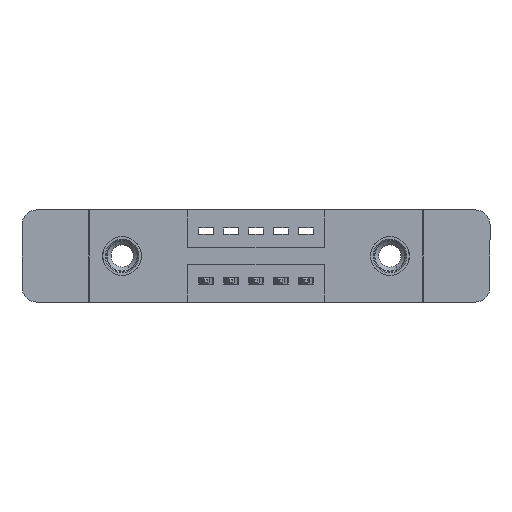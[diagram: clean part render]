
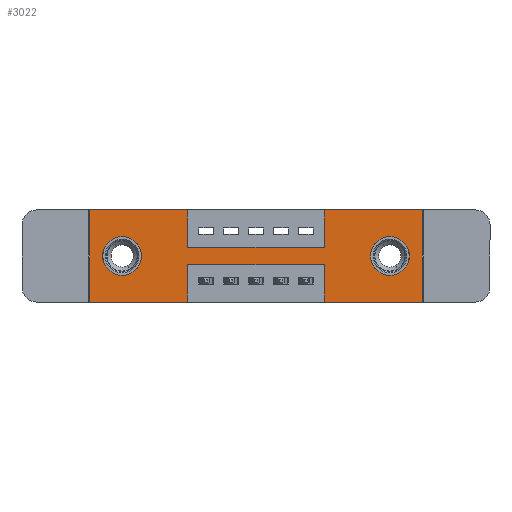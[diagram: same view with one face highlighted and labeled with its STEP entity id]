
A CAD part, front view. The second image highlights one B-rep face of the part: STEP entity #3022.
In plain terms, the highlighted planar face has unit normal (0, -1, 0).
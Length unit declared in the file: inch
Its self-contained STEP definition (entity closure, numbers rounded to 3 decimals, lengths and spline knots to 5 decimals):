
#40 = VECTOR ( 'NONE', #10457, 39.37008 ) ;
#335 = AXIS2_PLACEMENT_3D ( 'NONE', #2708, #11473, #4994 ) ;
#441 = VECTOR ( 'NONE', #3727, 39.37008 ) ;
#442 = VECTOR ( 'NONE', #2713, 39.37008 ) ;
#696 = EDGE_CURVE ( 'NONE', #11015, #10530, #4663, .T. ) ;
#732 = ORIENTED_EDGE ( 'NONE', *, *, #8910, .F. ) ;
#839 = LINE ( 'NONE', #7332, #11649 ) ;
#999 = CARTESIAN_POINT ( 'NONE',  ( 0., 0., -0.37 ) ) ;
#1172 = VECTOR ( 'NONE', #13573, 39.37008 ) ;
#1231 = EDGE_CURVE ( 'NONE', #11217, #7812, #3303, .T. ) ;
#1261 = VERTEX_POINT ( 'NONE', #6042 ) ;
#1301 = VERTEX_POINT ( 'NONE', #3097 ) ;
#1337 = ORIENTED_EDGE ( 'NONE', *, *, #5611, .F. ) ;
#1374 = CARTESIAN_POINT ( 'NONE',  ( 0.13, 0., -0.185 ) ) ;
#1427 = AXIS2_PLACEMENT_3D ( 'NONE', #5837, #6946, #1541 ) ;
#1432 = LINE ( 'NONE', #1782, #7557 ) ;
#1444 = LINE ( 'NONE', #6855, #441 ) ;
#1499 = DIRECTION ( 'NONE',  ( 0., 0., -1. ) ) ;
#1541 = DIRECTION ( 'NONE',  ( 0., 0., 1. ) ) ;
#1595 = DIRECTION ( 'NONE',  ( 0., 1., 0. ) ) ;
#1655 = EDGE_LOOP ( 'NONE', ( #13437, #12144, #732, #12489, #5523, #8941, #12088, #11838, #7246, #10654, #1337, #10598 ) ) ;
#1717 = VERTEX_POINT ( 'NONE', #11412 ) ;
#1782 = CARTESIAN_POINT ( 'NONE',  ( 0., 0., -0.37 ) ) ;
#2211 = LINE ( 'NONE', #9366, #40 ) ;
#2405 = CARTESIAN_POINT ( 'NONE',  ( 1.335, 0., 0. ) ) ;
#2530 = DIRECTION ( 'NONE',  ( 1., 0., 0. ) ) ;
#2640 = CARTESIAN_POINT ( 'NONE',  ( 0., 0., 0. ) ) ;
#2665 = ORIENTED_EDGE ( 'NONE', *, *, #8342, .T. ) ;
#2708 = CARTESIAN_POINT ( 'NONE',  ( 1.205, 0., -0.185 ) ) ;
#2713 = DIRECTION ( 'NONE',  ( 0., 0., -1. ) ) ;
#2794 = CARTESIAN_POINT ( 'NONE',  ( 1.335, 0., 0. ) ) ;
#2797 = VECTOR ( 'NONE', #5978, 39.37008 ) ;
#2984 = CIRCLE ( 'NONE', #1427, 0.078 ) ;
#3022 = ADVANCED_FACE ( 'NONE', ( #10549, #8697, #5294 ), #7953, .T. ) ;
#3045 = DIRECTION ( 'NONE',  ( -1., 0., 0. ) ) ;
#3097 = CARTESIAN_POINT ( 'NONE',  ( 0.13, 0., -0.263 ) ) ;
#3152 = CARTESIAN_POINT ( 'NONE',  ( 0.3925, 0., -0.15 ) ) ;
#3303 = LINE ( 'NONE', #7256, #442 ) ;
#3496 = CARTESIAN_POINT ( 'NONE',  ( 0., 0., 0. ) ) ;
#3504 = DIRECTION ( 'NONE',  ( 0., 0., 1. ) ) ;
#3627 = DIRECTION ( 'NONE',  ( 0., -1., 0. ) ) ;
#3727 = DIRECTION ( 'NONE',  ( 0., 0., 1. ) ) ;
#3757 = EDGE_CURVE ( 'NONE', #1717, #11015, #2211, .T. ) ;
#3911 = VERTEX_POINT ( 'NONE', #5735 ) ;
#4175 = CIRCLE ( 'NONE', #9367, 0.078 ) ;
#4194 = VERTEX_POINT ( 'NONE', #3496 ) ;
#4247 = CIRCLE ( 'NONE', #335, 0.078 ) ;
#4253 = VERTEX_POINT ( 'NONE', #9760 ) ;
#4655 = CARTESIAN_POINT ( 'NONE',  ( 0.3925, 0., 0. ) ) ;
#4663 = LINE ( 'NONE', #2640, #2797 ) ;
#4710 = CARTESIAN_POINT ( 'NONE',  ( 0., 0., -0.37 ) ) ;
#4851 = ORIENTED_EDGE ( 'NONE', *, *, #12152, .T. ) ;
#4985 = LINE ( 'NONE', #5798, #10904 ) ;
#4994 = DIRECTION ( 'NONE',  ( 0., 0., -1. ) ) ;
#5043 = EDGE_CURVE ( 'NONE', #12837, #11812, #12834, .T. ) ;
#5129 = EDGE_CURVE ( 'NONE', #4194, #12837, #5736, .T. ) ;
#5294 = FACE_OUTER_BOUND ( 'NONE', #1655, .T. ) ;
#5468 = CARTESIAN_POINT ( 'NONE',  ( 0.9425, 0., -0.22 ) ) ;
#5523 = ORIENTED_EDGE ( 'NONE', *, *, #10918, .F. ) ;
#5611 = EDGE_CURVE ( 'NONE', #9312, #4194, #10639, .T. ) ;
#5660 = CARTESIAN_POINT ( 'NONE',  ( 0., 0., 0. ) ) ;
#5677 = DIRECTION ( 'NONE',  ( 0., 1., 0. ) ) ;
#5735 = CARTESIAN_POINT ( 'NONE',  ( 0.13, 0., -0.107 ) ) ;
#5736 = LINE ( 'NONE', #5660, #1172 ) ;
#5768 = EDGE_CURVE ( 'NONE', #11917, #11217, #839, .T. ) ;
#5769 = CIRCLE ( 'NONE', #13616, 0.078 ) ;
#5798 = CARTESIAN_POINT ( 'NONE',  ( 0., 0., -0.37 ) ) ;
#5837 = CARTESIAN_POINT ( 'NONE',  ( 0.13, 0., -0.185 ) ) ;
#5940 = DIRECTION ( 'NONE',  ( -1., 0., 0. ) ) ;
#5978 = DIRECTION ( 'NONE',  ( 1., 0., 0. ) ) ;
#6042 = CARTESIAN_POINT ( 'NONE',  ( 1.205, 0., -0.107 ) ) ;
#6117 = EDGE_CURVE ( 'NONE', #11812, #1717, #10613, .T. ) ;
#6475 = LINE ( 'NONE', #2405, #7832 ) ;
#6645 = EDGE_LOOP ( 'NONE', ( #7209, #4851 ) ) ;
#6855 = CARTESIAN_POINT ( 'NONE',  ( 0.9425, 0., -0.37 ) ) ;
#6946 = DIRECTION ( 'NONE',  ( 0., 1., 0. ) ) ;
#7184 = CARTESIAN_POINT ( 'NONE',  ( 0.3925, 0., 0. ) ) ;
#7209 = ORIENTED_EDGE ( 'NONE', *, *, #12194, .T. ) ;
#7246 = ORIENTED_EDGE ( 'NONE', *, *, #5043, .F. ) ;
#7256 = CARTESIAN_POINT ( 'NONE',  ( 0.3925, 0., -0.37 ) ) ;
#7269 = VECTOR ( 'NONE', #2530, 39.37008 ) ;
#7329 = CARTESIAN_POINT ( 'NONE',  ( 0.3925, 0., -0.22 ) ) ;
#7332 = CARTESIAN_POINT ( 'NONE',  ( 0.3925, 0., -0.22 ) ) ;
#7557 = VECTOR ( 'NONE', #3045, 39.37008 ) ;
#7812 = VERTEX_POINT ( 'NONE', #9895 ) ;
#7832 = VECTOR ( 'NONE', #7916, 39.37008 ) ;
#7916 = DIRECTION ( 'NONE',  ( 0., 0., -1. ) ) ;
#7953 = PLANE ( 'NONE',  #13760 ) ;
#8005 = EDGE_CURVE ( 'NONE', #3911, #1301, #2984, .T. ) ;
#8216 = DIRECTION ( 'NONE',  ( 0., 0., 1. ) ) ;
#8342 = EDGE_CURVE ( 'NONE', #1301, #3911, #4175, .T. ) ;
#8553 = VERTEX_POINT ( 'NONE', #12533 ) ;
#8592 = VERTEX_POINT ( 'NONE', #13742 ) ;
#8697 = FACE_BOUND ( 'NONE', #10923, .T. ) ;
#8910 = EDGE_CURVE ( 'NONE', #8553, #11917, #1444, .T. ) ;
#8941 = ORIENTED_EDGE ( 'NONE', *, *, #696, .F. ) ;
#9126 = VECTOR ( 'NONE', #8216, 39.37008 ) ;
#9166 = CARTESIAN_POINT ( 'NONE',  ( 1.205, 0., -0.185 ) ) ;
#9194 = CARTESIAN_POINT ( 'NONE',  ( 0.9425, 0., 0. ) ) ;
#9295 = ORIENTED_EDGE ( 'NONE', *, *, #8005, .T. ) ;
#9312 = VERTEX_POINT ( 'NONE', #999 ) ;
#9339 = CARTESIAN_POINT ( 'NONE',  ( 0., 0., 0. ) ) ;
#9366 = CARTESIAN_POINT ( 'NONE',  ( 0.9425, 0., 0. ) ) ;
#9367 = AXIS2_PLACEMENT_3D ( 'NONE', #1374, #5677, #3504 ) ;
#9482 = EDGE_CURVE ( 'NONE', #4253, #8553, #4985, .T. ) ;
#9544 = EDGE_CURVE ( 'NONE', #7812, #9312, #1432, .T. ) ;
#9760 = CARTESIAN_POINT ( 'NONE',  ( 1.335, 0., -0.37 ) ) ;
#9895 = CARTESIAN_POINT ( 'NONE',  ( 0.3925, 0., -0.37 ) ) ;
#10119 = VECTOR ( 'NONE', #1499, 39.37008 ) ;
#10457 = DIRECTION ( 'NONE',  ( 0., 0., 1. ) ) ;
#10530 = VERTEX_POINT ( 'NONE', #2794 ) ;
#10549 = FACE_BOUND ( 'NONE', #6645, .T. ) ;
#10598 = ORIENTED_EDGE ( 'NONE', *, *, #9544, .F. ) ;
#10613 = LINE ( 'NONE', #11352, #7269 ) ;
#10639 = LINE ( 'NONE', #9339, #9126 ) ;
#10654 = ORIENTED_EDGE ( 'NONE', *, *, #5129, .F. ) ;
#10904 = VECTOR ( 'NONE', #5940, 39.37008 ) ;
#10918 = EDGE_CURVE ( 'NONE', #10530, #4253, #6475, .T. ) ;
#10923 = EDGE_LOOP ( 'NONE', ( #9295, #2665 ) ) ;
#11015 = VERTEX_POINT ( 'NONE', #9194 ) ;
#11205 = DIRECTION ( 'NONE',  ( 0., 0., -1. ) ) ;
#11217 = VERTEX_POINT ( 'NONE', #7329 ) ;
#11352 = CARTESIAN_POINT ( 'NONE',  ( 0.3925, 0., -0.15 ) ) ;
#11412 = CARTESIAN_POINT ( 'NONE',  ( 0.9425, 0., -0.15 ) ) ;
#11473 = DIRECTION ( 'NONE',  ( 0., 1., 0. ) ) ;
#11649 = VECTOR ( 'NONE', #13845, 39.37008 ) ;
#11812 = VERTEX_POINT ( 'NONE', #3152 ) ;
#11838 = ORIENTED_EDGE ( 'NONE', *, *, #6117, .F. ) ;
#11917 = VERTEX_POINT ( 'NONE', #5468 ) ;
#12088 = ORIENTED_EDGE ( 'NONE', *, *, #3757, .F. ) ;
#12144 = ORIENTED_EDGE ( 'NONE', *, *, #5768, .F. ) ;
#12152 = EDGE_CURVE ( 'NONE', #8592, #1261, #5769, .T. ) ;
#12194 = EDGE_CURVE ( 'NONE', #1261, #8592, #4247, .T. ) ;
#12403 = DIRECTION ( 'NONE',  ( 0., 0., -1. ) ) ;
#12489 = ORIENTED_EDGE ( 'NONE', *, *, #9482, .F. ) ;
#12533 = CARTESIAN_POINT ( 'NONE',  ( 0.9425, 0., -0.37 ) ) ;
#12834 = LINE ( 'NONE', #4655, #10119 ) ;
#12837 = VERTEX_POINT ( 'NONE', #7184 ) ;
#13437 = ORIENTED_EDGE ( 'NONE', *, *, #1231, .F. ) ;
#13573 = DIRECTION ( 'NONE',  ( 1., 0., 0. ) ) ;
#13616 = AXIS2_PLACEMENT_3D ( 'NONE', #9166, #1595, #12403 ) ;
#13742 = CARTESIAN_POINT ( 'NONE',  ( 1.205, 0., -0.263 ) ) ;
#13760 = AXIS2_PLACEMENT_3D ( 'NONE', #4710, #3627, #11205 ) ;
#13845 = DIRECTION ( 'NONE',  ( -1., 0., 0. ) ) ;
